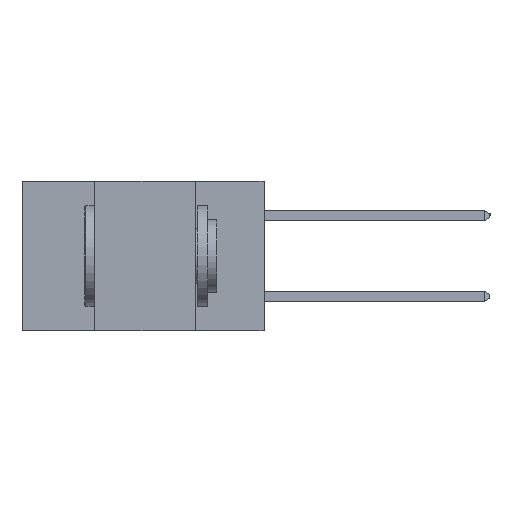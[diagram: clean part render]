
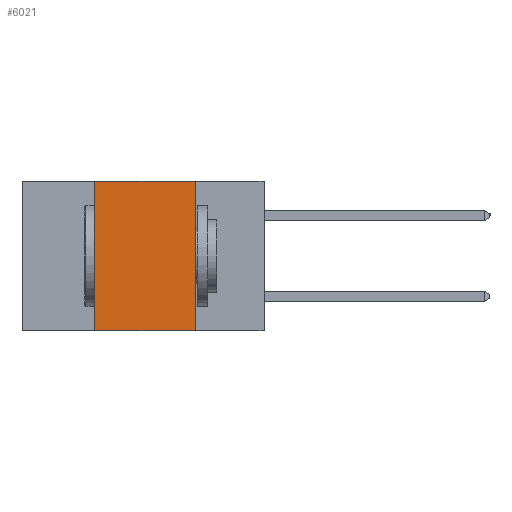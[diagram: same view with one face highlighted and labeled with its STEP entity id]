
A CAD part, left-side view. The second image highlights one B-rep face of the part: STEP entity #6021.
In plain terms, the highlighted planar face has unit normal (-1, 0, 0).
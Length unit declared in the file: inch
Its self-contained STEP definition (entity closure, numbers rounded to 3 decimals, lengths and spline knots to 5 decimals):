
#10 = CARTESIAN_POINT ( 'NONE',  ( 0., 0.17, 0. ) ) ;
#63 = PLANE ( 'NONE',  #610 ) ;
#610 = AXIS2_PLACEMENT_3D ( 'NONE', #12435, #4238, #17493 ) ;
#820 = CARTESIAN_POINT ( 'NONE',  ( 0., 0.42, -0.37 ) ) ;
#875 = VECTOR ( 'NONE', #4663, 39.37008 ) ;
#1139 = EDGE_CURVE ( 'NONE', #4352, #11695, #12485, .T. ) ;
#1528 = ORIENTED_EDGE ( 'NONE', *, *, #7504, .F. ) ;
#1678 = VECTOR ( 'NONE', #6974, 39.37008 ) ;
#2012 = ORIENTED_EDGE ( 'NONE', *, *, #1139, .T. ) ;
#2372 = CARTESIAN_POINT ( 'NONE',  ( 0., 0.42, 0. ) ) ;
#3222 = VERTEX_POINT ( 'NONE', #2372 ) ;
#4189 = VECTOR ( 'NONE', #13696, 39.37008 ) ;
#4238 = DIRECTION ( 'NONE',  ( 1., 0., 0. ) ) ;
#4352 = VERTEX_POINT ( 'NONE', #9623 ) ;
#4663 = DIRECTION ( 'NONE',  ( 0., -1., 0. ) ) ;
#6021 = ADVANCED_FACE ( 'NONE', ( #15880 ), #63, .F. ) ;
#6253 = DIRECTION ( 'NONE',  ( 0., 0., 1. ) ) ;
#6974 = DIRECTION ( 'NONE',  ( 0., -1., 0. ) ) ;
#7290 = EDGE_LOOP ( 'NONE', ( #8447, #1528, #11199, #2012 ) ) ;
#7504 = EDGE_CURVE ( 'NONE', #3222, #10552, #8864, .T. ) ;
#8447 = ORIENTED_EDGE ( 'NONE', *, *, #16700, .F. ) ;
#8609 = CARTESIAN_POINT ( 'NONE',  ( 0., 0.6, 0. ) ) ;
#8803 = EDGE_CURVE ( 'NONE', #4352, #3222, #13014, .T. ) ;
#8864 = LINE ( 'NONE', #8609, #875 ) ;
#8883 = VECTOR ( 'NONE', #6253, 39.37008 ) ;
#9623 = CARTESIAN_POINT ( 'NONE',  ( 0., 0.42, -0.37 ) ) ;
#10552 = VERTEX_POINT ( 'NONE', #10 ) ;
#10961 = CARTESIAN_POINT ( 'NONE',  ( 0., 0.17, -0.37 ) ) ;
#11199 = ORIENTED_EDGE ( 'NONE', *, *, #8803, .F. ) ;
#11695 = VERTEX_POINT ( 'NONE', #15837 ) ;
#12399 = CARTESIAN_POINT ( 'NONE',  ( 0., 0.6, -0.37 ) ) ;
#12435 = CARTESIAN_POINT ( 'NONE',  ( 0., 0.6, 0. ) ) ;
#12468 = LINE ( 'NONE', #10961, #4189 ) ;
#12485 = LINE ( 'NONE', #12399, #1678 ) ;
#13014 = LINE ( 'NONE', #820, #8883 ) ;
#13696 = DIRECTION ( 'NONE',  ( 0., 0., -1. ) ) ;
#15837 = CARTESIAN_POINT ( 'NONE',  ( 0., 0.17, -0.37 ) ) ;
#15880 = FACE_OUTER_BOUND ( 'NONE', #7290, .T. ) ;
#16700 = EDGE_CURVE ( 'NONE', #10552, #11695, #12468, .T. ) ;
#17493 = DIRECTION ( 'NONE',  ( 0., 0., -1. ) ) ;
